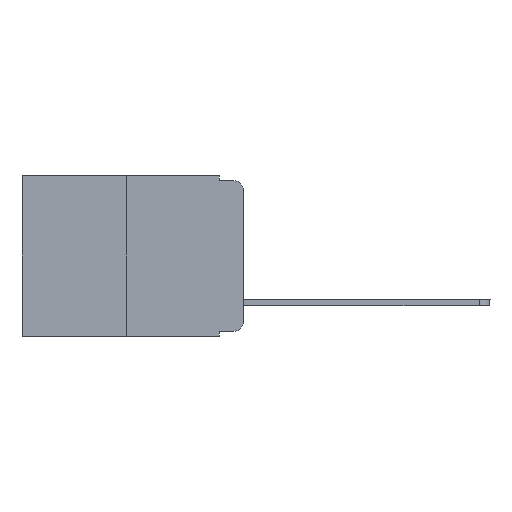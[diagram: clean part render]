
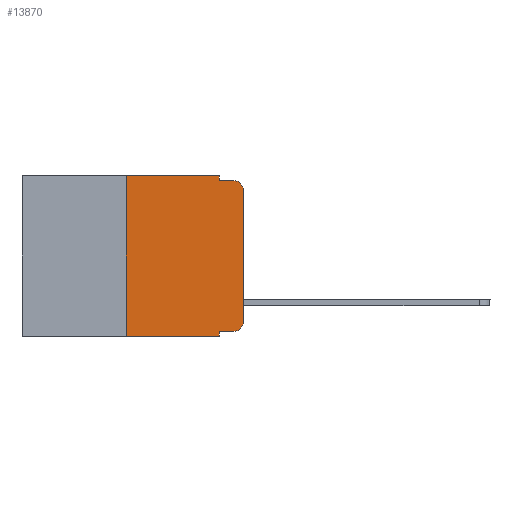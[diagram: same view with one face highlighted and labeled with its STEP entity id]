
A CAD part, left-side view. The second image highlights one B-rep face of the part: STEP entity #13870.
In plain terms, the highlighted planar face has unit normal (-1, 0, 0).
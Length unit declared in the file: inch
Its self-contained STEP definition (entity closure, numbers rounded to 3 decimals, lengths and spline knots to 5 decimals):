
#349 = CARTESIAN_POINT ( 'NONE',  ( 0., 0., -0.313 ) ) ;
#728 = ORIENTED_EDGE ( 'NONE', *, *, #16424, .T. ) ;
#866 = EDGE_CURVE ( 'NONE', #14827, #4605, #7520, .T. ) ;
#1146 = VECTOR ( 'NONE', #14990, 39.37008 ) ;
#1490 = CARTESIAN_POINT ( 'NONE',  ( 0., 0.25, -0.343 ) ) ;
#1529 = VECTOR ( 'NONE', #3340, 39.37008 ) ;
#1831 = ORIENTED_EDGE ( 'NONE', *, *, #866, .F. ) ;
#2418 = VECTOR ( 'NONE', #10231, 39.37008 ) ;
#3058 = PLANE ( 'NONE',  #14538 ) ;
#3340 = DIRECTION ( 'NONE',  ( 0., 0., 1. ) ) ;
#3655 = VERTEX_POINT ( 'NONE', #12582 ) ;
#3818 = CARTESIAN_POINT ( 'NONE',  ( 0., 0.25, 0. ) ) ;
#3926 = CARTESIAN_POINT ( 'NONE',  ( 0., 0.051, -0.333 ) ) ;
#4263 = EDGE_CURVE ( 'NONE', #4464, #14827, #4328, .T. ) ;
#4328 = LINE ( 'NONE', #14517, #15067 ) ;
#4464 = VERTEX_POINT ( 'NONE', #3818 ) ;
#4538 = DIRECTION ( 'NONE',  ( 0., 0., -1. ) ) ;
#4605 = VERTEX_POINT ( 'NONE', #12976 ) ;
#4613 = CARTESIAN_POINT ( 'NONE',  ( 0., 0.02, -0.01 ) ) ;
#4635 = CARTESIAN_POINT ( 'NONE',  ( 0., 0.25, 0. ) ) ;
#5539 = LINE ( 'NONE', #12613, #13390 ) ;
#6629 = EDGE_CURVE ( 'NONE', #4605, #8899, #6648, .T. ) ;
#6648 = LINE ( 'NONE', #6927, #18490 ) ;
#6927 = CARTESIAN_POINT ( 'NONE',  ( 0., 0.051, -0.01 ) ) ;
#7160 = CARTESIAN_POINT ( 'NONE',  ( 0., 0.473, 0. ) ) ;
#7200 = VERTEX_POINT ( 'NONE', #1490 ) ;
#7266 = VECTOR ( 'NONE', #10481, 39.37008 ) ;
#7520 = LINE ( 'NONE', #16611, #7266 ) ;
#7933 = EDGE_CURVE ( 'NONE', #9159, #13088, #5539, .T. ) ;
#8866 = VECTOR ( 'NONE', #16150, 39.37008 ) ;
#8879 = DIRECTION ( 'NONE',  ( 1., 0., 0. ) ) ;
#8899 = VERTEX_POINT ( 'NONE', #4613 ) ;
#9159 = VERTEX_POINT ( 'NONE', #3926 ) ;
#9917 = ORIENTED_EDGE ( 'NONE', *, *, #17526, .T. ) ;
#10157 = ORIENTED_EDGE ( 'NONE', *, *, #4263, .F. ) ;
#10216 = EDGE_CURVE ( 'NONE', #7200, #4464, #12253, .T. ) ;
#10231 = DIRECTION ( 'NONE',  ( 0., -1., 0. ) ) ;
#10481 = DIRECTION ( 'NONE',  ( 0., 0., -1. ) ) ;
#10913 = EDGE_LOOP ( 'NONE', ( #728, #9917, #11394, #1831, #10157, #15515, #14465, #15014, #17021, #18146 ) ) ;
#10961 = LINE ( 'NONE', #15322, #1529 ) ;
#11112 = DIRECTION ( 'NONE',  ( -1., 0., 0. ) ) ;
#11175 = DIRECTION ( 'NONE',  ( 0., -1., 0. ) ) ;
#11297 = CARTESIAN_POINT ( 'NONE',  ( 0., 0.02, -0.03 ) ) ;
#11394 = ORIENTED_EDGE ( 'NONE', *, *, #6629, .F. ) ;
#11654 = AXIS2_PLACEMENT_3D ( 'NONE', #11297, #11112, #14052 ) ;
#11836 = EDGE_CURVE ( 'NONE', #9159, #14209, #12443, .T. ) ;
#12010 = CIRCLE ( 'NONE', #11654, 0.02 ) ;
#12253 = LINE ( 'NONE', #4635, #8866 ) ;
#12443 = LINE ( 'NONE', #18103, #1146 ) ;
#12447 = CARTESIAN_POINT ( 'NONE',  ( 0., 0.02, -0.333 ) ) ;
#12569 = DIRECTION ( 'NONE',  ( 0., -1., 0. ) ) ;
#12582 = CARTESIAN_POINT ( 'NONE',  ( 0., 0., -0.03 ) ) ;
#12613 = CARTESIAN_POINT ( 'NONE',  ( 0., 0.051, -0.333 ) ) ;
#12927 = CARTESIAN_POINT ( 'NONE',  ( 0., 0.02, -0.313 ) ) ;
#12976 = CARTESIAN_POINT ( 'NONE',  ( 0., 0.051, -0.01 ) ) ;
#12982 = DIRECTION ( 'NONE',  ( 0., 0., -1. ) ) ;
#13088 = VERTEX_POINT ( 'NONE', #12447 ) ;
#13092 = LINE ( 'NONE', #17415, #2418 ) ;
#13390 = VECTOR ( 'NONE', #11175, 39.37008 ) ;
#13870 = ADVANCED_FACE ( 'NONE', ( #16095 ), #3058, .F. ) ;
#14052 = DIRECTION ( 'NONE',  ( 0., 0., -1. ) ) ;
#14209 = VERTEX_POINT ( 'NONE', #17372 ) ;
#14340 = DIRECTION ( 'NONE',  ( 0., -1., 0. ) ) ;
#14465 = ORIENTED_EDGE ( 'NONE', *, *, #15946, .T. ) ;
#14517 = CARTESIAN_POINT ( 'NONE',  ( 0., 0.473, 0. ) ) ;
#14538 = AXIS2_PLACEMENT_3D ( 'NONE', #7160, #8879, #12982 ) ;
#14827 = VERTEX_POINT ( 'NONE', #15348 ) ;
#14990 = DIRECTION ( 'NONE',  ( 0., 0., -1. ) ) ;
#15014 = ORIENTED_EDGE ( 'NONE', *, *, #11836, .F. ) ;
#15067 = VECTOR ( 'NONE', #14340, 39.37008 ) ;
#15322 = CARTESIAN_POINT ( 'NONE',  ( 0., 0., 0. ) ) ;
#15348 = CARTESIAN_POINT ( 'NONE',  ( 0., 0.051, 0. ) ) ;
#15515 = ORIENTED_EDGE ( 'NONE', *, *, #10216, .F. ) ;
#15916 = CIRCLE ( 'NONE', #18331, 0.02 ) ;
#15946 = EDGE_CURVE ( 'NONE', #7200, #14209, #13092, .T. ) ;
#16095 = FACE_OUTER_BOUND ( 'NONE', #10913, .T. ) ;
#16150 = DIRECTION ( 'NONE',  ( 0., 0., 1. ) ) ;
#16424 = EDGE_CURVE ( 'NONE', #17761, #3655, #10961, .T. ) ;
#16611 = CARTESIAN_POINT ( 'NONE',  ( 0., 0.051, 0. ) ) ;
#17021 = ORIENTED_EDGE ( 'NONE', *, *, #7933, .T. ) ;
#17199 = EDGE_CURVE ( 'NONE', #13088, #17761, #15916, .T. ) ;
#17372 = CARTESIAN_POINT ( 'NONE',  ( 0., 0.051, -0.343 ) ) ;
#17415 = CARTESIAN_POINT ( 'NONE',  ( 0., 0.473, -0.343 ) ) ;
#17446 = DIRECTION ( 'NONE',  ( -1., 0., 0. ) ) ;
#17526 = EDGE_CURVE ( 'NONE', #3655, #8899, #12010, .T. ) ;
#17761 = VERTEX_POINT ( 'NONE', #349 ) ;
#18103 = CARTESIAN_POINT ( 'NONE',  ( 0., 0.051, 0. ) ) ;
#18146 = ORIENTED_EDGE ( 'NONE', *, *, #17199, .T. ) ;
#18331 = AXIS2_PLACEMENT_3D ( 'NONE', #12927, #17446, #4538 ) ;
#18490 = VECTOR ( 'NONE', #12569, 39.37008 ) ;
